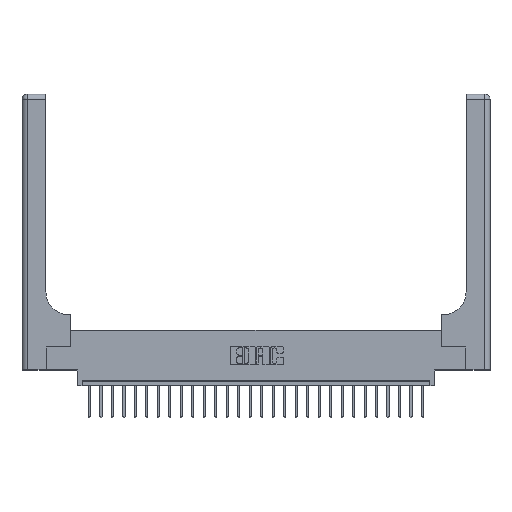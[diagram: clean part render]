
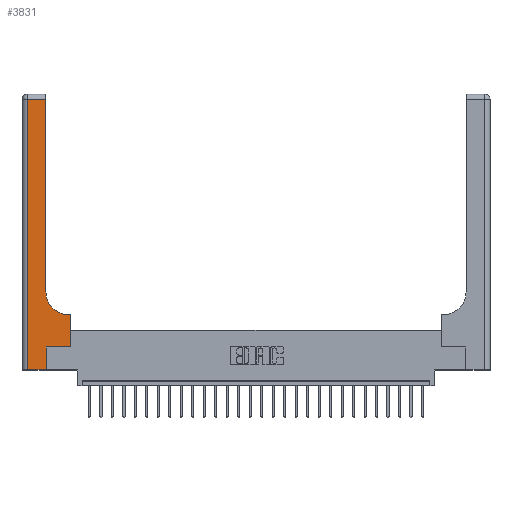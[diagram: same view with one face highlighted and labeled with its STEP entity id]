
A CAD part, top view. The second image highlights one B-rep face of the part: STEP entity #3831.
In plain terms, the highlighted planar face has unit normal (0, 0, 1).
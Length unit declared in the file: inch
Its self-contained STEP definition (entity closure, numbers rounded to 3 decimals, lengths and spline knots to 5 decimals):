
#1658 = FACE_OUTER_BOUND ( 'NONE', #7182, .T. ) ;
#1685 = CARTESIAN_POINT ( 'NONE',  ( 0.265, 0., 0.37 ) ) ;
#1881 = CARTESIAN_POINT ( 'NONE',  ( 0.51, 0.85, 0.37 ) ) ;
#2140 = CARTESIAN_POINT ( 'NONE',  ( 0.26, 2.94, 0.37 ) ) ;
#2275 = DIRECTION ( 'NONE',  ( -1., 0., 0. ) ) ;
#2288 = DIRECTION ( 'NONE',  ( 1., 0., 0. ) ) ;
#2907 = VECTOR ( 'NONE', #12289, 39.37008 ) ;
#2910 = VECTOR ( 'NONE', #11823, 39.37008 ) ;
#3221 = EDGE_CURVE ( 'NONE', #10741, #25233, #5268, .T. ) ;
#3434 = CARTESIAN_POINT ( 'NONE',  ( 0.06, 0., 0.37 ) ) ;
#3831 = ADVANCED_FACE ( 'NONE', ( #1658 ), #9695, .F. ) ;
#4729 = VECTOR ( 'NONE', #24478, 39.37008 ) ;
#5157 = EDGE_CURVE ( 'NONE', #24378, #10741, #15517, .T. ) ;
#5268 = LINE ( 'NONE', #13303, #18039 ) ;
#5300 = DIRECTION ( 'NONE',  ( -1., 0., 0. ) ) ;
#5824 = ORIENTED_EDGE ( 'NONE', *, *, #8689, .T. ) ;
#5986 = CARTESIAN_POINT ( 'NONE',  ( 0., 0., 0.37 ) ) ;
#6353 = VECTOR ( 'NONE', #2288, 39.37008 ) ;
#6745 = DIRECTION ( 'NONE',  ( 0., 1., 0. ) ) ;
#7059 = ORIENTED_EDGE ( 'NONE', *, *, #24302, .T. ) ;
#7182 = EDGE_LOOP ( 'NONE', ( #10310, #7059, #5824, #14215, #16688, #22134, #16378, #7652, #7350 ) ) ;
#7220 = DIRECTION ( 'NONE',  ( 1., 0., 0. ) ) ;
#7350 = ORIENTED_EDGE ( 'NONE', *, *, #5157, .T. ) ;
#7652 = ORIENTED_EDGE ( 'NONE', *, *, #9894, .T. ) ;
#7771 = CARTESIAN_POINT ( 'NONE',  ( 0.265, 0.25, 0.37 ) ) ;
#8201 = LINE ( 'NONE', #24107, #2907 ) ;
#8689 = EDGE_CURVE ( 'NONE', #10610, #11767, #12910, .T. ) ;
#9431 = DIRECTION ( 'NONE',  ( 0., 0., -1. ) ) ;
#9695 = PLANE ( 'NONE',  #24575 ) ;
#9894 = EDGE_CURVE ( 'NONE', #16365, #24378, #24370, .T. ) ;
#10310 = ORIENTED_EDGE ( 'NONE', *, *, #3221, .T. ) ;
#10489 = CARTESIAN_POINT ( 'NONE',  ( 0.06, 2.94, 0.37 ) ) ;
#10610 = VERTEX_POINT ( 'NONE', #10489 ) ;
#10741 = VERTEX_POINT ( 'NONE', #20604 ) ;
#11108 = EDGE_CURVE ( 'NONE', #15831, #16365, #8201, .T. ) ;
#11234 = LINE ( 'NONE', #23194, #24836 ) ;
#11767 = VERTEX_POINT ( 'NONE', #3434 ) ;
#11823 = DIRECTION ( 'NONE',  ( 0., 1., 0. ) ) ;
#12016 = EDGE_CURVE ( 'NONE', #21951, #15831, #25781, .T. ) ;
#12138 = CARTESIAN_POINT ( 'NONE',  ( 0.528, 0.25, 0.37 ) ) ;
#12203 = LINE ( 'NONE', #1685, #2910 ) ;
#12289 = DIRECTION ( 'NONE',  ( 0., 1., 0. ) ) ;
#12910 = LINE ( 'NONE', #18714, #4729 ) ;
#13303 = CARTESIAN_POINT ( 'NONE',  ( 0.26, 3., 0.37 ) ) ;
#13852 = EDGE_CURVE ( 'NONE', #14623, #21951, #12203, .T. ) ;
#14060 = CARTESIAN_POINT ( 'NONE',  ( 0.265, 0.25, 0.37 ) ) ;
#14215 = ORIENTED_EDGE ( 'NONE', *, *, #24010, .T. ) ;
#14328 = DIRECTION ( 'NONE',  ( 1., 0., 0. ) ) ;
#14526 = DIRECTION ( 'NONE',  ( -1., 0., 0. ) ) ;
#14623 = VERTEX_POINT ( 'NONE', #17933 ) ;
#15050 = VECTOR ( 'NONE', #14328, 39.37008 ) ;
#15517 = CIRCLE ( 'NONE', #20135, 0.25 ) ;
#15831 = VERTEX_POINT ( 'NONE', #12138 ) ;
#15984 = LINE ( 'NONE', #5986, #6353 ) ;
#16243 = DIRECTION ( 'NONE',  ( 0., 0., -1. ) ) ;
#16365 = VERTEX_POINT ( 'NONE', #19577 ) ;
#16378 = ORIENTED_EDGE ( 'NONE', *, *, #11108, .T. ) ;
#16688 = ORIENTED_EDGE ( 'NONE', *, *, #13852, .T. ) ;
#17545 = CARTESIAN_POINT ( 'NONE',  ( 0.51, 0.6, 0.37 ) ) ;
#17933 = CARTESIAN_POINT ( 'NONE',  ( 0.265, 0., 0.37 ) ) ;
#18039 = VECTOR ( 'NONE', #6745, 39.37008 ) ;
#18714 = CARTESIAN_POINT ( 'NONE',  ( 0.06, 3., 0.37 ) ) ;
#19577 = CARTESIAN_POINT ( 'NONE',  ( 0.528, 0.6, 0.37 ) ) ;
#20135 = AXIS2_PLACEMENT_3D ( 'NONE', #1881, #9431, #7220 ) ;
#20604 = CARTESIAN_POINT ( 'NONE',  ( 0.26, 0.85, 0.37 ) ) ;
#21951 = VERTEX_POINT ( 'NONE', #14060 ) ;
#22134 = ORIENTED_EDGE ( 'NONE', *, *, #12016, .T. ) ;
#22268 = CARTESIAN_POINT ( 'NONE',  ( 0.26, 0.6, 0.37 ) ) ;
#22823 = VECTOR ( 'NONE', #2275, 39.37008 ) ;
#23194 = CARTESIAN_POINT ( 'NONE',  ( 0., 2.94, 0.37 ) ) ;
#24010 = EDGE_CURVE ( 'NONE', #11767, #14623, #15984, .T. ) ;
#24107 = CARTESIAN_POINT ( 'NONE',  ( 0.528, 0.25, 0.37 ) ) ;
#24302 = EDGE_CURVE ( 'NONE', #25233, #10610, #11234, .T. ) ;
#24370 = LINE ( 'NONE', #22268, #22823 ) ;
#24378 = VERTEX_POINT ( 'NONE', #17545 ) ;
#24478 = DIRECTION ( 'NONE',  ( 0., -1., 0. ) ) ;
#24575 = AXIS2_PLACEMENT_3D ( 'NONE', #25732, #16243, #14526 ) ;
#24836 = VECTOR ( 'NONE', #5300, 39.37008 ) ;
#25233 = VERTEX_POINT ( 'NONE', #2140 ) ;
#25732 = CARTESIAN_POINT ( 'NONE',  ( 0., 3., 0.37 ) ) ;
#25781 = LINE ( 'NONE', #7771, #15050 ) ;
